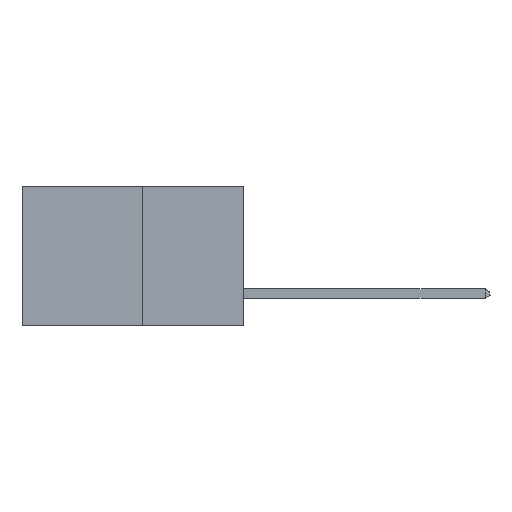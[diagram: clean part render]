
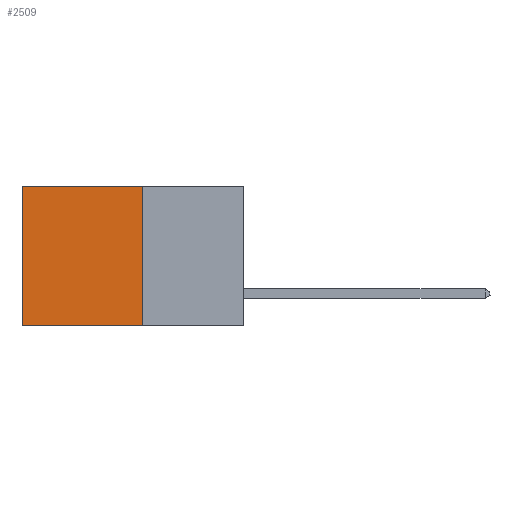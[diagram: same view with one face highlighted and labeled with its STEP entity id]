
A CAD part, left-side view. The second image highlights one B-rep face of the part: STEP entity #2509.
In plain terms, the highlighted planar face has unit normal (-1, 0, 0).
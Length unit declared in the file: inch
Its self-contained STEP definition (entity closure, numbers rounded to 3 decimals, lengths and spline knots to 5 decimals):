
#646 = CARTESIAN_POINT ( 'NONE',  ( 0.277, 0.27, -0.37 ) ) ;
#672 = DIRECTION ( 'NONE',  ( 1., 0., 0. ) ) ;
#711 = DIRECTION ( 'NONE',  ( 0., 0., -1. ) ) ;
#796 = FACE_OUTER_BOUND ( 'NONE', #6799, .T. ) ;
#809 = PLANE ( 'NONE',  #2620 ) ;
#986 = EDGE_CURVE ( 'NONE', #4119, #4281, #2887, .T. ) ;
#1442 = CARTESIAN_POINT ( 'NONE',  ( 0.277, 0.59, -0.37 ) ) ;
#1511 = EDGE_CURVE ( 'NONE', #2232, #4119, #9124, .T. ) ;
#2232 = VERTEX_POINT ( 'NONE', #9198 ) ;
#2509 = ADVANCED_FACE ( 'NONE', ( #796 ), #809, .F. ) ;
#2554 = CARTESIAN_POINT ( 'NONE',  ( 0.277, 0.27, -0.37 ) ) ;
#2578 = VECTOR ( 'NONE', #3732, 39.37008 ) ;
#2620 = AXIS2_PLACEMENT_3D ( 'NONE', #646, #672, #711 ) ;
#2824 = ORIENTED_EDGE ( 'NONE', *, *, #5238, .T. ) ;
#2839 = ORIENTED_EDGE ( 'NONE', *, *, #986, .F. ) ;
#2850 = ORIENTED_EDGE ( 'NONE', *, *, #1511, .F. ) ;
#2857 = VECTOR ( 'NONE', #6766, 39.37008 ) ;
#2887 = LINE ( 'NONE', #7501, #7135 ) ;
#2890 = ORIENTED_EDGE ( 'NONE', *, *, #10167, .T. ) ;
#2907 = VERTEX_POINT ( 'NONE', #8001 ) ;
#3732 = DIRECTION ( 'NONE',  ( 0., 0., -1. ) ) ;
#3945 = CARTESIAN_POINT ( 'NONE',  ( 0.277, 0.59, -0.37 ) ) ;
#4119 = VERTEX_POINT ( 'NONE', #2554 ) ;
#4281 = VERTEX_POINT ( 'NONE', #1442 ) ;
#5238 = EDGE_CURVE ( 'NONE', #2907, #4281, #10635, .T. ) ;
#5284 = VECTOR ( 'NONE', #8495, 39.37008 ) ;
#6766 = DIRECTION ( 'NONE',  ( 0., 0., -1. ) ) ;
#6799 = EDGE_LOOP ( 'NONE', ( #2824, #2839, #2850, #2890 ) ) ;
#6978 = CARTESIAN_POINT ( 'NONE',  ( 0.277, 0.27, 0. ) ) ;
#7135 = VECTOR ( 'NONE', #7515, 39.37008 ) ;
#7501 = CARTESIAN_POINT ( 'NONE',  ( 0.277, 0.27, -0.37 ) ) ;
#7515 = DIRECTION ( 'NONE',  ( 0., 1., 0. ) ) ;
#7518 = LINE ( 'NONE', #6978, #5284 ) ;
#8001 = CARTESIAN_POINT ( 'NONE',  ( 0.277, 0.59, 0. ) ) ;
#8495 = DIRECTION ( 'NONE',  ( 0., 1., 0. ) ) ;
#9124 = LINE ( 'NONE', #10442, #2857 ) ;
#9198 = CARTESIAN_POINT ( 'NONE',  ( 0.277, 0.27, 0. ) ) ;
#10167 = EDGE_CURVE ( 'NONE', #2232, #2907, #7518, .T. ) ;
#10442 = CARTESIAN_POINT ( 'NONE',  ( 0.277, 0.27, -0.37 ) ) ;
#10635 = LINE ( 'NONE', #3945, #2578 ) ;
